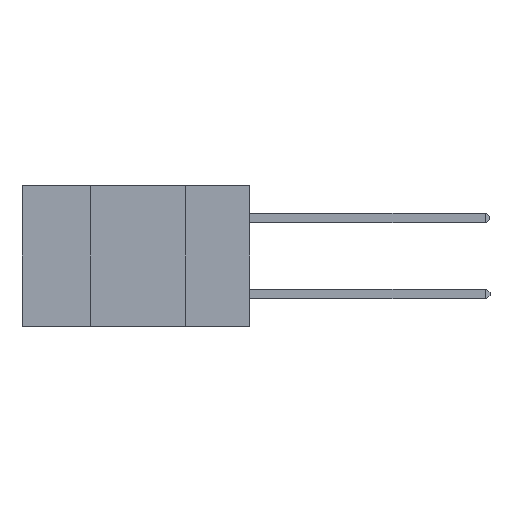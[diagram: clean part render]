
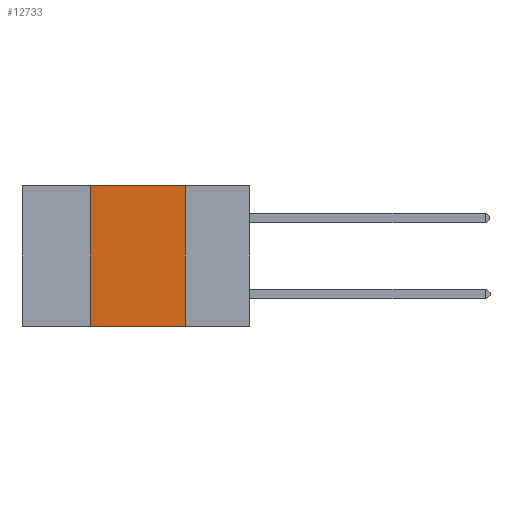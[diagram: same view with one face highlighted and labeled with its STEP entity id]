
A CAD part, left-side view. The second image highlights one B-rep face of the part: STEP entity #12733.
In plain terms, the highlighted planar face has unit normal (-1, 0, 0).
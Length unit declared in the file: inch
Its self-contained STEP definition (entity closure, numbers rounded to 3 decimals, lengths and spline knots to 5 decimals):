
#1219 = CARTESIAN_POINT ( 'NONE',  ( 0., 0.42, 0. ) ) ;
#1403 = LINE ( 'NONE', #16524, #19469 ) ;
#2005 = ORIENTED_EDGE ( 'NONE', *, *, #7548, .F. ) ;
#2230 = CARTESIAN_POINT ( 'NONE',  ( 0., 0.42, -0.37 ) ) ;
#3228 = VERTEX_POINT ( 'NONE', #12919 ) ;
#3328 = ORIENTED_EDGE ( 'NONE', *, *, #15971, .F. ) ;
#3729 = VECTOR ( 'NONE', #8531, 39.37008 ) ;
#4721 = CARTESIAN_POINT ( 'NONE',  ( 0., 0.17, 0. ) ) ;
#6157 = DIRECTION ( 'NONE',  ( 0., -1., 0. ) ) ;
#6235 = EDGE_CURVE ( 'NONE', #17685, #3228, #1403, .T. ) ;
#6581 = DIRECTION ( 'NONE',  ( 0., 0., -1. ) ) ;
#7548 = EDGE_CURVE ( 'NONE', #18175, #22408, #16843, .T. ) ;
#7667 = PLANE ( 'NONE',  #17827 ) ;
#8531 = DIRECTION ( 'NONE',  ( 0., 0., 1. ) ) ;
#8827 = VECTOR ( 'NONE', #6581, 39.37008 ) ;
#9482 = ORIENTED_EDGE ( 'NONE', *, *, #19269, .F. ) ;
#10752 = CARTESIAN_POINT ( 'NONE',  ( 0., 0.42, 0. ) ) ;
#11116 = CARTESIAN_POINT ( 'NONE',  ( 0., 0.17, 0. ) ) ;
#11223 = DIRECTION ( 'NONE',  ( 0., 0., -1. ) ) ;
#11594 = CARTESIAN_POINT ( 'NONE',  ( 0., 0.6, 0. ) ) ;
#11838 = EDGE_LOOP ( 'NONE', ( #9482, #2005, #3328, #16502 ) ) ;
#12733 = ADVANCED_FACE ( 'NONE', ( #20608 ), #7667, .F. ) ;
#12911 = VECTOR ( 'NONE', #15034, 39.37008 ) ;
#12919 = CARTESIAN_POINT ( 'NONE',  ( 0., 0.17, -0.37 ) ) ;
#15034 = DIRECTION ( 'NONE',  ( 0., -1., 0. ) ) ;
#15971 = EDGE_CURVE ( 'NONE', #17685, #18175, #20961, .T. ) ;
#16502 = ORIENTED_EDGE ( 'NONE', *, *, #6235, .T. ) ;
#16524 = CARTESIAN_POINT ( 'NONE',  ( 0., 0.6, -0.37 ) ) ;
#16843 = LINE ( 'NONE', #11594, #12911 ) ;
#17685 = VERTEX_POINT ( 'NONE', #2230 ) ;
#17827 = AXIS2_PLACEMENT_3D ( 'NONE', #19582, #21238, #11223 ) ;
#18175 = VERTEX_POINT ( 'NONE', #10752 ) ;
#19269 = EDGE_CURVE ( 'NONE', #22408, #3228, #22278, .T. ) ;
#19469 = VECTOR ( 'NONE', #6157, 39.37008 ) ;
#19582 = CARTESIAN_POINT ( 'NONE',  ( 0., 0.6, 0. ) ) ;
#20608 = FACE_OUTER_BOUND ( 'NONE', #11838, .T. ) ;
#20961 = LINE ( 'NONE', #1219, #3729 ) ;
#21238 = DIRECTION ( 'NONE',  ( 1., 0., 0. ) ) ;
#22278 = LINE ( 'NONE', #4721, #8827 ) ;
#22408 = VERTEX_POINT ( 'NONE', #11116 ) ;
